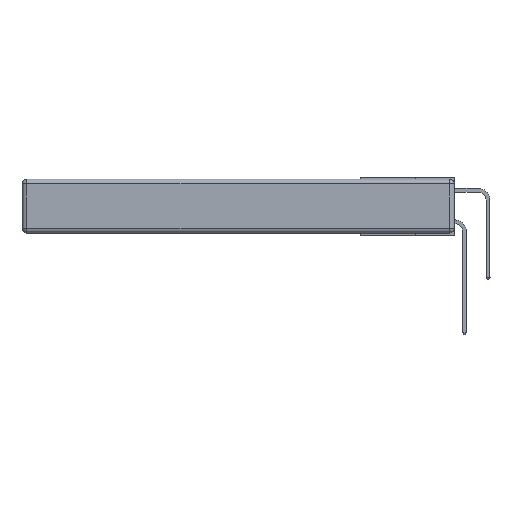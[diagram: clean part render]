
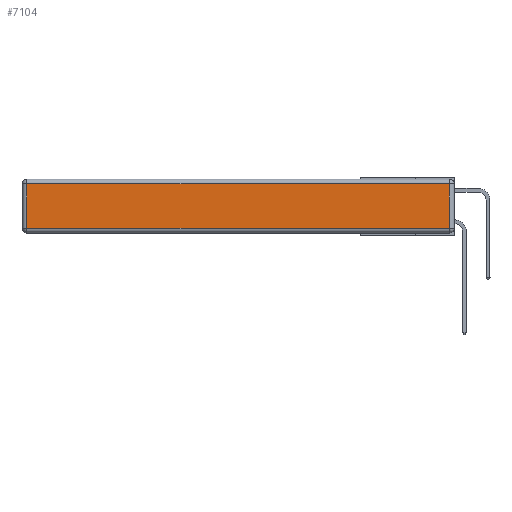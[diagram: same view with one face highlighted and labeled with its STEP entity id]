
A CAD part, left-side view. The second image highlights one B-rep face of the part: STEP entity #7104.
In plain terms, the highlighted planar face has unit normal (-1, 0, 0).
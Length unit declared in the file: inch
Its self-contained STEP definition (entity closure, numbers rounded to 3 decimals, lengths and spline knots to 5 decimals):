
#651 = VERTEX_POINT ( 'NONE', #7808 ) ;
#738 = DIRECTION ( 'NONE',  ( 0., 0., 1. ) ) ;
#1663 = EDGE_CURVE ( 'NONE', #7312, #651, #15569, .T. ) ;
#1716 = VECTOR ( 'NONE', #13579, 39.37008 ) ;
#2168 = AXIS2_PLACEMENT_3D ( 'NONE', #7408, #8597, #13590 ) ;
#2247 = ORIENTED_EDGE ( 'NONE', *, *, #14499, .T. ) ;
#2290 = ORIENTED_EDGE ( 'NONE', *, *, #9740, .T. ) ;
#3826 = PLANE ( 'NONE',  #2168 ) ;
#4455 = VECTOR ( 'NONE', #14884, 39.37008 ) ;
#5528 = VECTOR ( 'NONE', #11847, 39.37008 ) ;
#5993 = EDGE_LOOP ( 'NONE', ( #2247, #11370, #11765, #2290 ) ) ;
#6407 = VERTEX_POINT ( 'NONE', #11669 ) ;
#6481 = LINE ( 'NONE', #6854, #10323 ) ;
#6854 = CARTESIAN_POINT ( 'NONE',  ( 0., 0.03, -0.343 ) ) ;
#6980 = CARTESIAN_POINT ( 'NONE',  ( 0., 0., -0.313 ) ) ;
#7104 = ADVANCED_FACE ( 'NONE', ( #7662 ), #3826, .T. ) ;
#7312 = VERTEX_POINT ( 'NONE', #9310 ) ;
#7408 = CARTESIAN_POINT ( 'NONE',  ( 0., 0., -0.343 ) ) ;
#7662 = FACE_OUTER_BOUND ( 'NONE', #5993, .T. ) ;
#7808 = CARTESIAN_POINT ( 'NONE',  ( 0., 2.72, -0.03 ) ) ;
#8356 = EDGE_CURVE ( 'NONE', #6407, #7312, #6481, .T. ) ;
#8597 = DIRECTION ( 'NONE',  ( -1., 0., 0. ) ) ;
#9310 = CARTESIAN_POINT ( 'NONE',  ( 0., 0.03, -0.03 ) ) ;
#9621 = CARTESIAN_POINT ( 'NONE',  ( 0., 2.72, -0.313 ) ) ;
#9740 = EDGE_CURVE ( 'NONE', #651, #11257, #10862, .T. ) ;
#10323 = VECTOR ( 'NONE', #738, 39.37008 ) ;
#10862 = LINE ( 'NONE', #13537, #1716 ) ;
#11257 = VERTEX_POINT ( 'NONE', #9621 ) ;
#11370 = ORIENTED_EDGE ( 'NONE', *, *, #8356, .T. ) ;
#11669 = CARTESIAN_POINT ( 'NONE',  ( 0., 0.03, -0.313 ) ) ;
#11765 = ORIENTED_EDGE ( 'NONE', *, *, #1663, .T. ) ;
#11847 = DIRECTION ( 'NONE',  ( 0., -1., 0. ) ) ;
#12832 = LINE ( 'NONE', #6980, #5528 ) ;
#13537 = CARTESIAN_POINT ( 'NONE',  ( 0., 2.72, -0.343 ) ) ;
#13579 = DIRECTION ( 'NONE',  ( 0., 0., -1. ) ) ;
#13590 = DIRECTION ( 'NONE',  ( 0., 0., 1. ) ) ;
#13758 = CARTESIAN_POINT ( 'NONE',  ( 0., 2.75, -0.03 ) ) ;
#14499 = EDGE_CURVE ( 'NONE', #11257, #6407, #12832, .T. ) ;
#14884 = DIRECTION ( 'NONE',  ( 0., 1., 0. ) ) ;
#15569 = LINE ( 'NONE', #13758, #4455 ) ;
